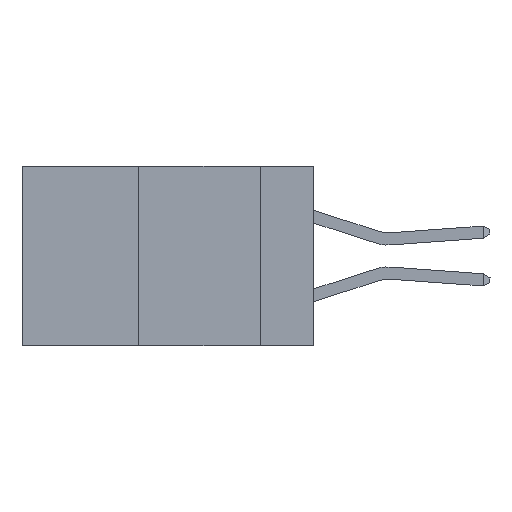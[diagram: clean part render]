
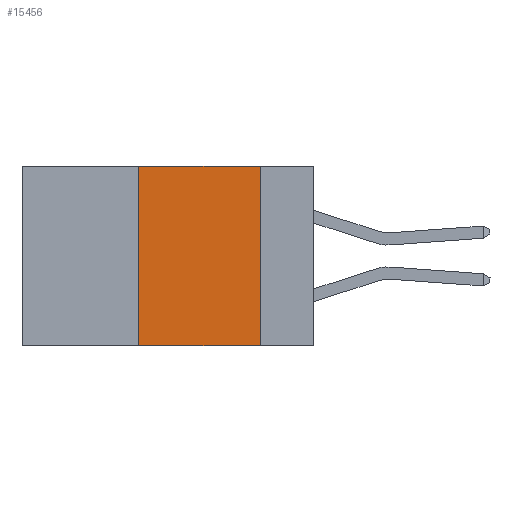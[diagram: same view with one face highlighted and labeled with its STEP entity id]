
A CAD part, left-side view. The second image highlights one B-rep face of the part: STEP entity #15456.
In plain terms, the highlighted planar face has unit normal (-1, 0, 0).
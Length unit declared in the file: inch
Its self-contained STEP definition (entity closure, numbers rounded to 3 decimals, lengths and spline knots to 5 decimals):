
#435 = LINE ( 'NONE', #3848, #7355 ) ;
#549 = VERTEX_POINT ( 'NONE', #8744 ) ;
#721 = DIRECTION ( 'NONE',  ( 0., 0., 1. ) ) ;
#3828 = CARTESIAN_POINT ( 'NONE',  ( 0., 0.6, 0. ) ) ;
#3848 = CARTESIAN_POINT ( 'NONE',  ( 0., 0.11, 0. ) ) ;
#4327 = VERTEX_POINT ( 'NONE', #6419 ) ;
#5193 = DIRECTION ( 'NONE',  ( 0., 0., -1. ) ) ;
#6038 = DIRECTION ( 'NONE',  ( 0., -1., 0. ) ) ;
#6412 = EDGE_CURVE ( 'NONE', #16900, #549, #10500, .T. ) ;
#6419 = CARTESIAN_POINT ( 'NONE',  ( 0., 0.36, -0.37 ) ) ;
#7355 = VECTOR ( 'NONE', #14040, 39.37008 ) ;
#8023 = VECTOR ( 'NONE', #10570, 39.37008 ) ;
#8084 = VECTOR ( 'NONE', #6038, 39.37008 ) ;
#8744 = CARTESIAN_POINT ( 'NONE',  ( 0., 0.11, 0. ) ) ;
#9669 = VECTOR ( 'NONE', #721, 39.37008 ) ;
#10237 = PLANE ( 'NONE',  #12273 ) ;
#10500 = LINE ( 'NONE', #10559, #8023 ) ;
#10559 = CARTESIAN_POINT ( 'NONE',  ( 0., 0.6, 0. ) ) ;
#10570 = DIRECTION ( 'NONE',  ( 0., -1., 0. ) ) ;
#11069 = VERTEX_POINT ( 'NONE', #14133 ) ;
#12225 = CARTESIAN_POINT ( 'NONE',  ( 0., 0.6, -0.37 ) ) ;
#12273 = AXIS2_PLACEMENT_3D ( 'NONE', #3828, #12684, #5193 ) ;
#12684 = DIRECTION ( 'NONE',  ( 1., 0., 0. ) ) ;
#12892 = EDGE_CURVE ( 'NONE', #4327, #16900, #12900, .T. ) ;
#12900 = LINE ( 'NONE', #13706, #9669 ) ;
#12995 = EDGE_CURVE ( 'NONE', #549, #11069, #435, .T. ) ;
#13293 = CARTESIAN_POINT ( 'NONE',  ( 0., 0.36, 0. ) ) ;
#13706 = CARTESIAN_POINT ( 'NONE',  ( 0., 0.36, 0. ) ) ;
#13949 = EDGE_LOOP ( 'NONE', ( #16815, #15961, #16626, #16391 ) ) ;
#14040 = DIRECTION ( 'NONE',  ( 0., 0., -1. ) ) ;
#14133 = CARTESIAN_POINT ( 'NONE',  ( 0., 0.11, -0.37 ) ) ;
#14245 = LINE ( 'NONE', #12225, #8084 ) ;
#14500 = EDGE_CURVE ( 'NONE', #4327, #11069, #14245, .T. ) ;
#15456 = ADVANCED_FACE ( 'NONE', ( #16456 ), #10237, .F. ) ;
#15961 = ORIENTED_EDGE ( 'NONE', *, *, #6412, .F. ) ;
#16391 = ORIENTED_EDGE ( 'NONE', *, *, #14500, .T. ) ;
#16456 = FACE_OUTER_BOUND ( 'NONE', #13949, .T. ) ;
#16626 = ORIENTED_EDGE ( 'NONE', *, *, #12892, .F. ) ;
#16815 = ORIENTED_EDGE ( 'NONE', *, *, #12995, .F. ) ;
#16900 = VERTEX_POINT ( 'NONE', #13293 ) ;
